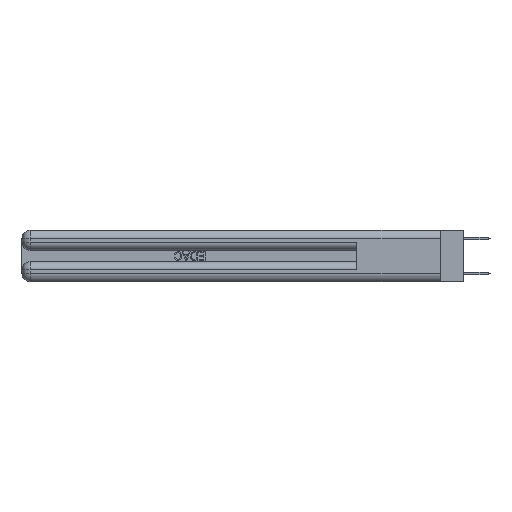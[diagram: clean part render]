
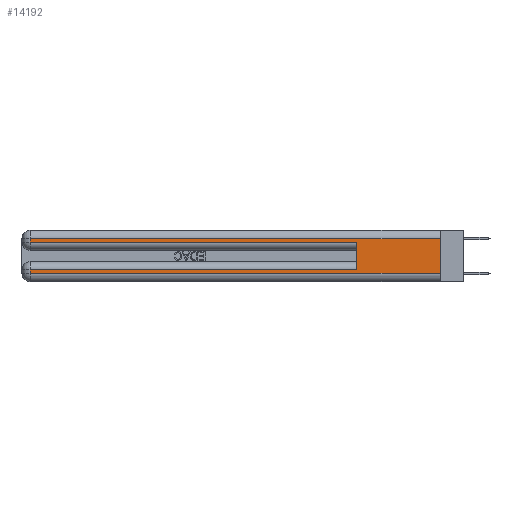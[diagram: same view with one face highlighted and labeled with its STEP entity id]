
A CAD part, left-side view. The second image highlights one B-rep face of the part: STEP entity #14192.
In plain terms, the highlighted planar face has unit normal (-1, 0, 0).
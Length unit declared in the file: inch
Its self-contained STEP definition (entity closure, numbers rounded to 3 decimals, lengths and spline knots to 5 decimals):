
#724 = CARTESIAN_POINT ( 'NONE',  ( 0., 2.94, 0.31 ) ) ;
#1348 = ORIENTED_EDGE ( 'NONE', *, *, #12389, .T. ) ;
#2093 = VECTOR ( 'NONE', #10577, 39.37008 ) ;
#2713 = DIRECTION ( 'NONE',  ( 0., 1., 0. ) ) ;
#3684 = VERTEX_POINT ( 'NONE', #35826 ) ;
#3937 = LINE ( 'NONE', #15332, #18322 ) ;
#4146 = LINE ( 'NONE', #15715, #18579 ) ;
#4492 = DIRECTION ( 'NONE',  ( 0., -1., 0. ) ) ;
#4585 = VERTEX_POINT ( 'NONE', #20800 ) ;
#4780 = CARTESIAN_POINT ( 'NONE',  ( 0., 0., 0.06 ) ) ;
#4822 = LINE ( 'NONE', #27630, #18239 ) ;
#4864 = VERTEX_POINT ( 'NONE', #26494 ) ;
#5140 = DIRECTION ( 'NONE',  ( 0., 0., -1. ) ) ;
#5606 = ORIENTED_EDGE ( 'NONE', *, *, #21521, .T. ) ;
#7736 = CARTESIAN_POINT ( 'NONE',  ( 0., 0., 0.31 ) ) ;
#7890 = ORIENTED_EDGE ( 'NONE', *, *, #30245, .F. ) ;
#7922 = VERTEX_POINT ( 'NONE', #36506 ) ;
#8293 = EDGE_CURVE ( 'NONE', #23835, #4585, #4146, .T. ) ;
#8474 = PLANE ( 'NONE',  #10517 ) ;
#8895 = VECTOR ( 'NONE', #2713, 39.37008 ) ;
#9531 = VECTOR ( 'NONE', #5140, 39.37008 ) ;
#10517 = AXIS2_PLACEMENT_3D ( 'NONE', #20418, #31852, #29056 ) ;
#10577 = DIRECTION ( 'NONE',  ( 0., -1., 0. ) ) ;
#11925 = CARTESIAN_POINT ( 'NONE',  ( 0., 0., 0.06 ) ) ;
#12389 = EDGE_CURVE ( 'NONE', #3684, #17911, #18984, .T. ) ;
#12689 = LINE ( 'NONE', #21097, #9531 ) ;
#12883 = LINE ( 'NONE', #16219, #20943 ) ;
#13152 = EDGE_CURVE ( 'NONE', #23762, #17911, #4822, .T. ) ;
#13690 = DIRECTION ( 'NONE',  ( 0., 0., -1. ) ) ;
#14192 = ADVANCED_FACE ( 'NONE', ( #28679 ), #8474, .F. ) ;
#15332 = CARTESIAN_POINT ( 'NONE',  ( 0., 0.6, 0.145 ) ) ;
#15715 = CARTESIAN_POINT ( 'NONE',  ( 0., 0., 0.285 ) ) ;
#16219 = CARTESIAN_POINT ( 'NONE',  ( 0., 0., 0.085 ) ) ;
#17911 = VERTEX_POINT ( 'NONE', #11925 ) ;
#17950 = DIRECTION ( 'NONE',  ( 0., 0., 1. ) ) ;
#18239 = VECTOR ( 'NONE', #24831, 39.37008 ) ;
#18322 = VECTOR ( 'NONE', #17950, 39.37008 ) ;
#18579 = VECTOR ( 'NONE', #4492, 39.37008 ) ;
#18949 = CARTESIAN_POINT ( 'NONE',  ( 0., 2.94, 0.285 ) ) ;
#18984 = LINE ( 'NONE', #4780, #2093 ) ;
#19042 = EDGE_CURVE ( 'NONE', #23762, #25032, #25321, .T. ) ;
#19848 = ORIENTED_EDGE ( 'NONE', *, *, #8293, .T. ) ;
#20191 = EDGE_CURVE ( 'NONE', #25032, #23835, #12689, .T. ) ;
#20418 = CARTESIAN_POINT ( 'NONE',  ( 0., 0., 0.37 ) ) ;
#20800 = CARTESIAN_POINT ( 'NONE',  ( 0., 0.6, 0.285 ) ) ;
#20943 = VECTOR ( 'NONE', #30463, 39.37008 ) ;
#21097 = CARTESIAN_POINT ( 'NONE',  ( 0., 2.94, 0.37 ) ) ;
#21521 = EDGE_CURVE ( 'NONE', #7922, #4864, #12883, .T. ) ;
#21756 = ORIENTED_EDGE ( 'NONE', *, *, #35348, .T. ) ;
#21879 = EDGE_LOOP ( 'NONE', ( #35563, #30396, #25104, #19848, #7890, #5606, #21756, #1348 ) ) ;
#22092 = CARTESIAN_POINT ( 'NONE',  ( 0., 2.94, 0.37 ) ) ;
#23762 = VERTEX_POINT ( 'NONE', #7736 ) ;
#23835 = VERTEX_POINT ( 'NONE', #18949 ) ;
#24831 = DIRECTION ( 'NONE',  ( 0., 0., -1. ) ) ;
#25032 = VERTEX_POINT ( 'NONE', #724 ) ;
#25104 = ORIENTED_EDGE ( 'NONE', *, *, #20191, .T. ) ;
#25321 = LINE ( 'NONE', #28326, #8895 ) ;
#26494 = CARTESIAN_POINT ( 'NONE',  ( 0., 2.94, 0.085 ) ) ;
#27630 = CARTESIAN_POINT ( 'NONE',  ( 0., 0., 0.37 ) ) ;
#28326 = CARTESIAN_POINT ( 'NONE',  ( 0., 0., 0.31 ) ) ;
#28679 = FACE_OUTER_BOUND ( 'NONE', #21879, .T. ) ;
#29056 = DIRECTION ( 'NONE',  ( 0., 0., -1. ) ) ;
#29502 = VECTOR ( 'NONE', #13690, 39.37008 ) ;
#30245 = EDGE_CURVE ( 'NONE', #7922, #4585, #3937, .T. ) ;
#30396 = ORIENTED_EDGE ( 'NONE', *, *, #19042, .T. ) ;
#30463 = DIRECTION ( 'NONE',  ( 0., 1., 0. ) ) ;
#30910 = LINE ( 'NONE', #22092, #29502 ) ;
#31852 = DIRECTION ( 'NONE',  ( 1., 0., 0. ) ) ;
#35348 = EDGE_CURVE ( 'NONE', #4864, #3684, #30910, .T. ) ;
#35563 = ORIENTED_EDGE ( 'NONE', *, *, #13152, .F. ) ;
#35826 = CARTESIAN_POINT ( 'NONE',  ( 0., 2.94, 0.06 ) ) ;
#36506 = CARTESIAN_POINT ( 'NONE',  ( 0., 0.6, 0.085 ) ) ;
